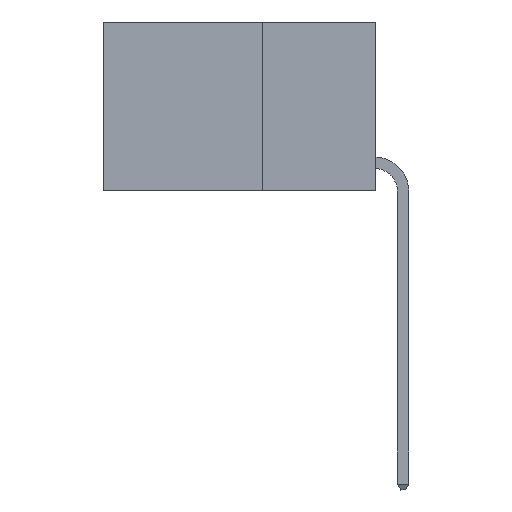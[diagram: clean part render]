
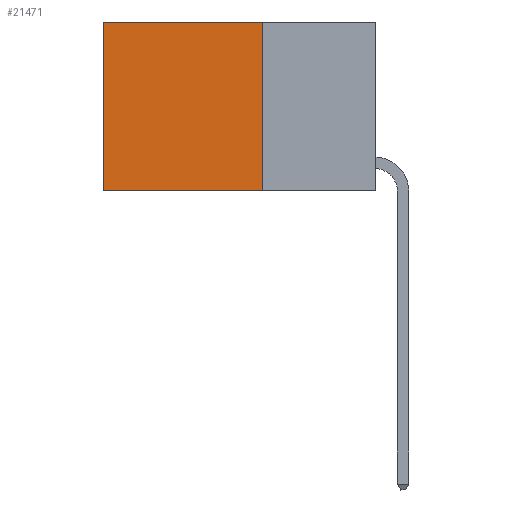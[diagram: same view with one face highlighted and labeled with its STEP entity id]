
A CAD part, left-side view. The second image highlights one B-rep face of the part: STEP entity #21471.
In plain terms, the highlighted planar face has unit normal (-1, 0, 0).
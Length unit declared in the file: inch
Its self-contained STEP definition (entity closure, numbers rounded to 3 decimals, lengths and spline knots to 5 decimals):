
#328 = DIRECTION ( 'NONE',  ( 1., 0., 0. ) ) ;
#329 = ORIENTED_EDGE ( 'NONE', *, *, #7636, .T. ) ;
#668 = VERTEX_POINT ( 'NONE', #14533 ) ;
#1773 = CARTESIAN_POINT ( 'NONE',  ( 0.2625, 0.25, -0.37 ) ) ;
#1807 = VECTOR ( 'NONE', #17762, 39.37008 ) ;
#2237 = LINE ( 'NONE', #19602, #10289 ) ;
#2573 = ORIENTED_EDGE ( 'NONE', *, *, #14361, .F. ) ;
#3196 = ORIENTED_EDGE ( 'NONE', *, *, #18197, .T. ) ;
#4408 = PLANE ( 'NONE',  #6328 ) ;
#6328 = AXIS2_PLACEMENT_3D ( 'NONE', #14111, #328, #20656 ) ;
#7190 = VERTEX_POINT ( 'NONE', #13197 ) ;
#7636 = EDGE_CURVE ( 'NONE', #19655, #7190, #2237, .T. ) ;
#7684 = CARTESIAN_POINT ( 'NONE',  ( 0.2625, 0.25, 0. ) ) ;
#8005 = CARTESIAN_POINT ( 'NONE',  ( 0.2625, 0.25, 0. ) ) ;
#10256 = VERTEX_POINT ( 'NONE', #1773 ) ;
#10289 = VECTOR ( 'NONE', #20223, 39.37008 ) ;
#10462 = FACE_OUTER_BOUND ( 'NONE', #11025, .T. ) ;
#10821 = CARTESIAN_POINT ( 'NONE',  ( 0.2625, 0.25, -0.37 ) ) ;
#11025 = EDGE_LOOP ( 'NONE', ( #3196, #11337, #2573, #329 ) ) ;
#11185 = LINE ( 'NONE', #10821, #13745 ) ;
#11337 = ORIENTED_EDGE ( 'NONE', *, *, #18233, .F. ) ;
#13014 = LINE ( 'NONE', #25174, #22118 ) ;
#13197 = CARTESIAN_POINT ( 'NONE',  ( 0.2625, 0.6, 0. ) ) ;
#13745 = VECTOR ( 'NONE', #19195, 39.37008 ) ;
#14111 = CARTESIAN_POINT ( 'NONE',  ( 0.2625, 0.25, 0. ) ) ;
#14361 = EDGE_CURVE ( 'NONE', #19655, #10256, #22059, .T. ) ;
#14533 = CARTESIAN_POINT ( 'NONE',  ( 0.2625, 0.6, -0.37 ) ) ;
#17762 = DIRECTION ( 'NONE',  ( 0., 0., -1. ) ) ;
#18197 = EDGE_CURVE ( 'NONE', #7190, #668, #13014, .T. ) ;
#18233 = EDGE_CURVE ( 'NONE', #10256, #668, #11185, .T. ) ;
#19195 = DIRECTION ( 'NONE',  ( 0., 1., 0. ) ) ;
#19602 = CARTESIAN_POINT ( 'NONE',  ( 0.2625, 0.25, 0. ) ) ;
#19655 = VERTEX_POINT ( 'NONE', #8005 ) ;
#20223 = DIRECTION ( 'NONE',  ( 0., 1., 0. ) ) ;
#20656 = DIRECTION ( 'NONE',  ( 0., 0., -1. ) ) ;
#21263 = DIRECTION ( 'NONE',  ( 0., 0., -1. ) ) ;
#21471 = ADVANCED_FACE ( 'NONE', ( #10462 ), #4408, .F. ) ;
#22059 = LINE ( 'NONE', #7684, #1807 ) ;
#22118 = VECTOR ( 'NONE', #21263, 39.37008 ) ;
#25174 = CARTESIAN_POINT ( 'NONE',  ( 0.2625, 0.6, 0. ) ) ;
